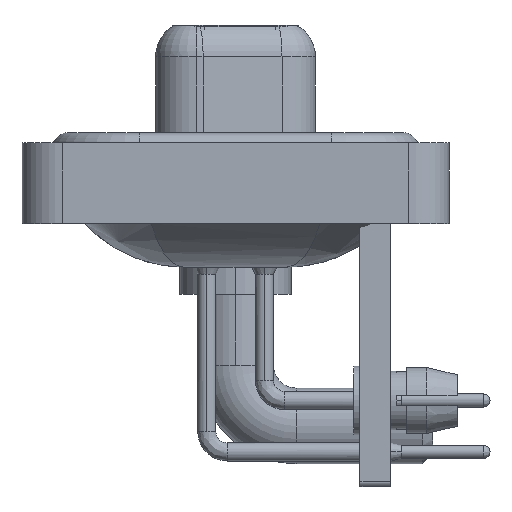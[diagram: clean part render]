
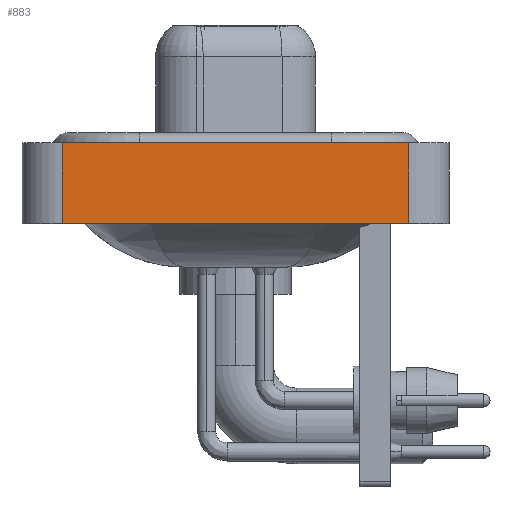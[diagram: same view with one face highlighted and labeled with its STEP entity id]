
A CAD part, left-side view. The second image highlights one B-rep face of the part: STEP entity #883.
In plain terms, the highlighted planar face has unit normal (-1, 0, 0).
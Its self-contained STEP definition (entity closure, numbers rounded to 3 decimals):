
#28 = CARTESIAN_POINT ( 'NONE',  ( -7.3, -8.55, -3.6 ) ) ;
#883 = ADVANCED_FACE ( 'NONE', ( #3512 ), #17165, .T. ) ;
#1065 = LINE ( 'NONE', #16485, #22394 ) ;
#1474 = ORIENTED_EDGE ( 'NONE', *, *, #4822, .T. ) ;
#1869 = EDGE_CURVE ( 'NONE', #14136, #23429, #1065, .T. ) ;
#3512 = FACE_OUTER_BOUND ( 'NONE', #20760, .T. ) ;
#3816 = LINE ( 'NONE', #3938, #17027 ) ;
#3938 = CARTESIAN_POINT ( 'NONE',  ( -7.3, 8.55, -3.6 ) ) ;
#4822 = EDGE_CURVE ( 'NONE', #22530, #23429, #9838, .T. ) ;
#4835 = ORIENTED_EDGE ( 'NONE', *, *, #10049, .F. ) ;
#5388 = CARTESIAN_POINT ( 'NONE',  ( -7.3, -8.55, -3.6 ) ) ;
#6063 = DIRECTION ( 'NONE',  ( 0., 0., 1. ) ) ;
#6831 = DIRECTION ( 'NONE',  ( 0., -1., 0. ) ) ;
#8072 = DIRECTION ( 'NONE',  ( 0., 0., 1. ) ) ;
#9838 = LINE ( 'NONE', #10224, #15718 ) ;
#10049 = EDGE_CURVE ( 'NONE', #20522, #14136, #3816, .T. ) ;
#10224 = CARTESIAN_POINT ( 'NONE',  ( -7.3, -8.55, -3.6 ) ) ;
#10293 = AXIS2_PLACEMENT_3D ( 'NONE', #5388, #18914, #11400 ) ;
#11400 = DIRECTION ( 'NONE',  ( 0., 0., 1. ) ) ;
#14136 = VERTEX_POINT ( 'NONE', #24136 ) ;
#15568 = ORIENTED_EDGE ( 'NONE', *, *, #1869, .F. ) ;
#15718 = VECTOR ( 'NONE', #8072, 1000. ) ;
#16485 = CARTESIAN_POINT ( 'NONE',  ( -7.3, -8.55, 0.4 ) ) ;
#16760 = CARTESIAN_POINT ( 'NONE',  ( -7.3, 8.55, -3.6 ) ) ;
#17027 = VECTOR ( 'NONE', #6063, 1000. ) ;
#17165 = PLANE ( 'NONE',  #10293 ) ;
#18914 = DIRECTION ( 'NONE',  ( -1., 0., 0. ) ) ;
#19542 = VECTOR ( 'NONE', #22089, 1000. ) ;
#20522 = VERTEX_POINT ( 'NONE', #16760 ) ;
#20760 = EDGE_LOOP ( 'NONE', ( #1474, #15568, #4835, #23146 ) ) ;
#21096 = CARTESIAN_POINT ( 'NONE',  ( -7.3, -8.55, 0.4 ) ) ;
#22089 = DIRECTION ( 'NONE',  ( 0., -1., 0. ) ) ;
#22294 = EDGE_CURVE ( 'NONE', #20522, #22530, #23848, .T. ) ;
#22394 = VECTOR ( 'NONE', #6831, 1000. ) ;
#22530 = VERTEX_POINT ( 'NONE', #28 ) ;
#23146 = ORIENTED_EDGE ( 'NONE', *, *, #22294, .T. ) ;
#23429 = VERTEX_POINT ( 'NONE', #21096 ) ;
#23737 = CARTESIAN_POINT ( 'NONE',  ( -7.3, -8.55, -3.6 ) ) ;
#23848 = LINE ( 'NONE', #23737, #19542 ) ;
#24136 = CARTESIAN_POINT ( 'NONE',  ( -7.3, 8.55, 0.4 ) ) ;
